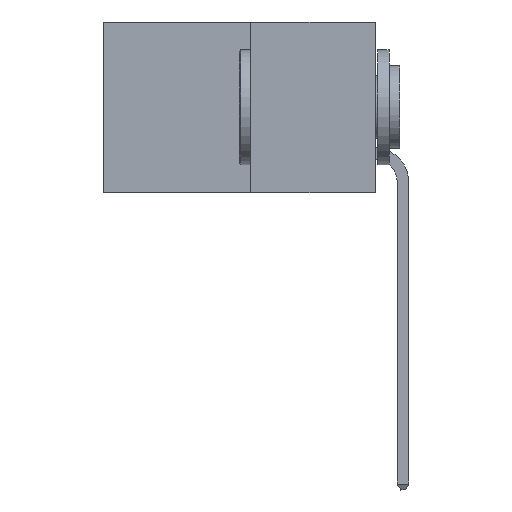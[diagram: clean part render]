
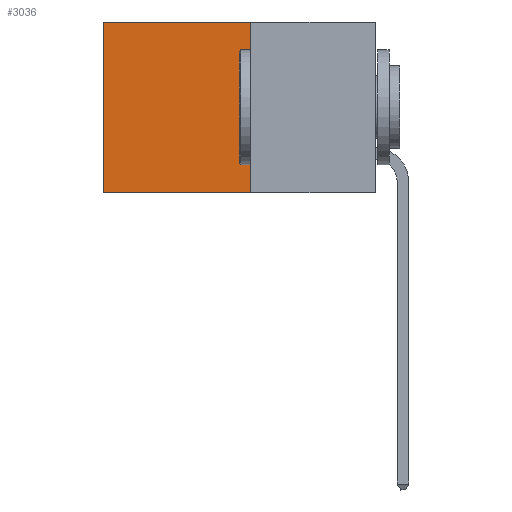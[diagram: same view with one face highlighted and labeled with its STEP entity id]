
A CAD part, left-side view. The second image highlights one B-rep face of the part: STEP entity #3036.
In plain terms, the highlighted planar face has unit normal (-1, 0, 0).
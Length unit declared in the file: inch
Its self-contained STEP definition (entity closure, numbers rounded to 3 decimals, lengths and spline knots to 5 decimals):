
#293 = ORIENTED_EDGE ( 'NONE', *, *, #505, .T. ) ;
#396 = VECTOR ( 'NONE', #11513, 39.37008 ) ;
#442 = CARTESIAN_POINT ( 'NONE',  ( 0.277, 0.27, -0.37 ) ) ;
#505 = EDGE_CURVE ( 'NONE', #8824, #10025, #4504, .T. ) ;
#607 = CARTESIAN_POINT ( 'NONE',  ( 0.277, 0.27, 0. ) ) ;
#1019 = AXIS2_PLACEMENT_3D ( 'NONE', #3385, #4340, #10973 ) ;
#1291 = CARTESIAN_POINT ( 'NONE',  ( 0.277, 0.59, -0.37 ) ) ;
#1598 = EDGE_CURVE ( 'NONE', #10025, #5454, #4946, .T. ) ;
#1767 = CARTESIAN_POINT ( 'NONE',  ( 0.277, 0.27, -0.37 ) ) ;
#2429 = PLANE ( 'NONE',  #1019 ) ;
#3036 = ADVANCED_FACE ( 'NONE', ( #4167 ), #2429, .F. ) ;
#3226 = EDGE_CURVE ( 'NONE', #3508, #5454, #7174, .T. ) ;
#3385 = CARTESIAN_POINT ( 'NONE',  ( 0.277, 0.27, -0.37 ) ) ;
#3508 = VERTEX_POINT ( 'NONE', #10642 ) ;
#3729 = EDGE_CURVE ( 'NONE', #8824, #3508, #11538, .T. ) ;
#3807 = CARTESIAN_POINT ( 'NONE',  ( 0.277, 0.59, 0. ) ) ;
#4167 = FACE_OUTER_BOUND ( 'NONE', #7804, .T. ) ;
#4241 = ORIENTED_EDGE ( 'NONE', *, *, #3729, .F. ) ;
#4312 = VECTOR ( 'NONE', #8457, 39.37008 ) ;
#4340 = DIRECTION ( 'NONE',  ( 1., 0., 0. ) ) ;
#4504 = LINE ( 'NONE', #607, #6759 ) ;
#4946 = LINE ( 'NONE', #9618, #396 ) ;
#5454 = VERTEX_POINT ( 'NONE', #1291 ) ;
#5742 = ORIENTED_EDGE ( 'NONE', *, *, #3226, .F. ) ;
#6759 = VECTOR ( 'NONE', #10697, 39.37008 ) ;
#7078 = ORIENTED_EDGE ( 'NONE', *, *, #1598, .T. ) ;
#7174 = LINE ( 'NONE', #1767, #4312 ) ;
#7192 = DIRECTION ( 'NONE',  ( 0., 0., -1. ) ) ;
#7804 = EDGE_LOOP ( 'NONE', ( #7078, #5742, #4241, #293 ) ) ;
#8457 = DIRECTION ( 'NONE',  ( 0., 1., 0. ) ) ;
#8824 = VERTEX_POINT ( 'NONE', #9387 ) ;
#9375 = VECTOR ( 'NONE', #7192, 39.37008 ) ;
#9387 = CARTESIAN_POINT ( 'NONE',  ( 0.277, 0.27, 0. ) ) ;
#9618 = CARTESIAN_POINT ( 'NONE',  ( 0.277, 0.59, -0.37 ) ) ;
#10025 = VERTEX_POINT ( 'NONE', #3807 ) ;
#10642 = CARTESIAN_POINT ( 'NONE',  ( 0.277, 0.27, -0.37 ) ) ;
#10697 = DIRECTION ( 'NONE',  ( 0., 1., 0. ) ) ;
#10973 = DIRECTION ( 'NONE',  ( 0., 0., -1. ) ) ;
#11513 = DIRECTION ( 'NONE',  ( 0., 0., -1. ) ) ;
#11538 = LINE ( 'NONE', #442, #9375 ) ;
